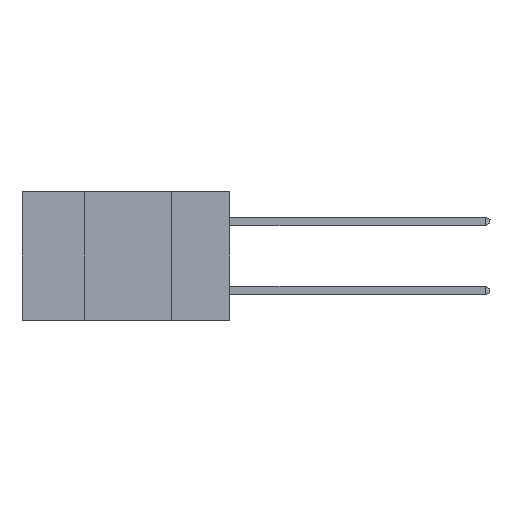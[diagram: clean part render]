
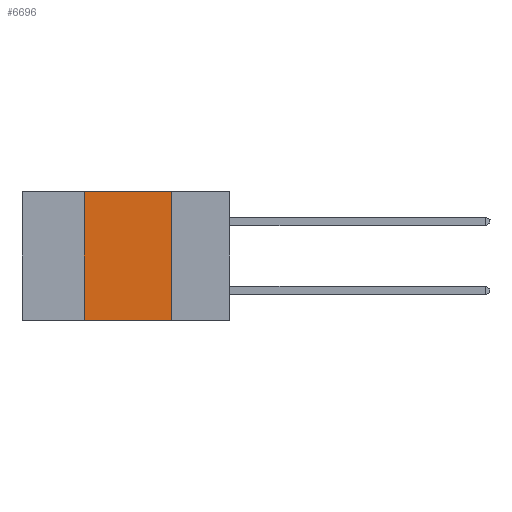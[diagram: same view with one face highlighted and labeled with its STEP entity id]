
A CAD part, left-side view. The second image highlights one B-rep face of the part: STEP entity #6696.
In plain terms, the highlighted planar face has unit normal (-1, 0, 0).
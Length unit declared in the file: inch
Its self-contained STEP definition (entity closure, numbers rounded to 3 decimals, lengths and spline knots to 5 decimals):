
#1074 = DIRECTION ( 'NONE',  ( 0., -1., 0. ) ) ;
#1284 = VERTEX_POINT ( 'NONE', #2376 ) ;
#1816 = ORIENTED_EDGE ( 'NONE', *, *, #14795, .F. ) ;
#2376 = CARTESIAN_POINT ( 'NONE',  ( 0., 0.17, -0.37 ) ) ;
#2440 = VECTOR ( 'NONE', #1074, 39.37008 ) ;
#2585 = CARTESIAN_POINT ( 'NONE',  ( 0., 0.42, 0. ) ) ;
#3033 = DIRECTION ( 'NONE',  ( 0., 0., -1. ) ) ;
#5186 = VERTEX_POINT ( 'NONE', #21081 ) ;
#5248 = CARTESIAN_POINT ( 'NONE',  ( 0., 0.6, 0. ) ) ;
#5344 = PLANE ( 'NONE',  #20624 ) ;
#5474 = DIRECTION ( 'NONE',  ( 1., 0., 0. ) ) ;
#6696 = ADVANCED_FACE ( 'NONE', ( #8973 ), #5344, .F. ) ;
#6871 = VECTOR ( 'NONE', #13475, 39.37008 ) ;
#7349 = CARTESIAN_POINT ( 'NONE',  ( 0., 0.6, -0.37 ) ) ;
#7524 = ORIENTED_EDGE ( 'NONE', *, *, #26054, .T. ) ;
#8973 = FACE_OUTER_BOUND ( 'NONE', #22356, .T. ) ;
#9052 = ORIENTED_EDGE ( 'NONE', *, *, #19614, .F. ) ;
#10217 = CARTESIAN_POINT ( 'NONE',  ( 0., 0.42, -0.37 ) ) ;
#11277 = CARTESIAN_POINT ( 'NONE',  ( 0., 0.6, 0. ) ) ;
#12624 = ORIENTED_EDGE ( 'NONE', *, *, #16561, .F. ) ;
#13475 = DIRECTION ( 'NONE',  ( 0., -1., 0. ) ) ;
#14795 = EDGE_CURVE ( 'NONE', #23179, #5186, #23257, .T. ) ;
#15314 = DIRECTION ( 'NONE',  ( 0., 0., -1. ) ) ;
#15914 = VECTOR ( 'NONE', #19361, 39.37008 ) ;
#16561 = EDGE_CURVE ( 'NONE', #20411, #23179, #17348, .T. ) ;
#17348 = LINE ( 'NONE', #25780, #15914 ) ;
#19021 = VECTOR ( 'NONE', #3033, 39.37008 ) ;
#19361 = DIRECTION ( 'NONE',  ( 0., 0., 1. ) ) ;
#19614 = EDGE_CURVE ( 'NONE', #5186, #1284, #21676, .T. ) ;
#20411 = VERTEX_POINT ( 'NONE', #10217 ) ;
#20624 = AXIS2_PLACEMENT_3D ( 'NONE', #11277, #5474, #15314 ) ;
#21081 = CARTESIAN_POINT ( 'NONE',  ( 0., 0.17, 0. ) ) ;
#21276 = CARTESIAN_POINT ( 'NONE',  ( 0., 0.17, -0.37 ) ) ;
#21676 = LINE ( 'NONE', #21276, #19021 ) ;
#21988 = LINE ( 'NONE', #7349, #2440 ) ;
#22356 = EDGE_LOOP ( 'NONE', ( #9052, #1816, #12624, #7524 ) ) ;
#23179 = VERTEX_POINT ( 'NONE', #2585 ) ;
#23257 = LINE ( 'NONE', #5248, #6871 ) ;
#25780 = CARTESIAN_POINT ( 'NONE',  ( 0., 0.42, -0.37 ) ) ;
#26054 = EDGE_CURVE ( 'NONE', #20411, #1284, #21988, .T. ) ;
